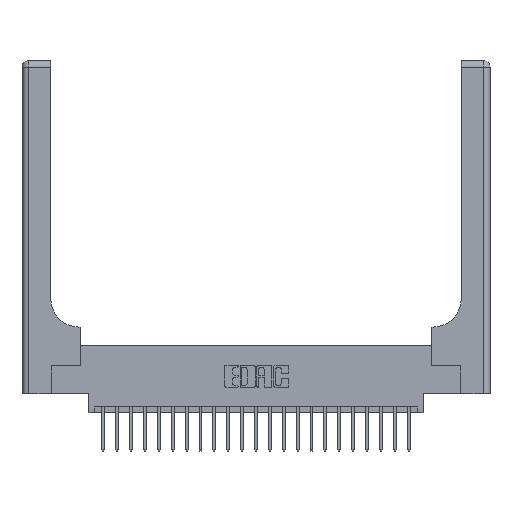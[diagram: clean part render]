
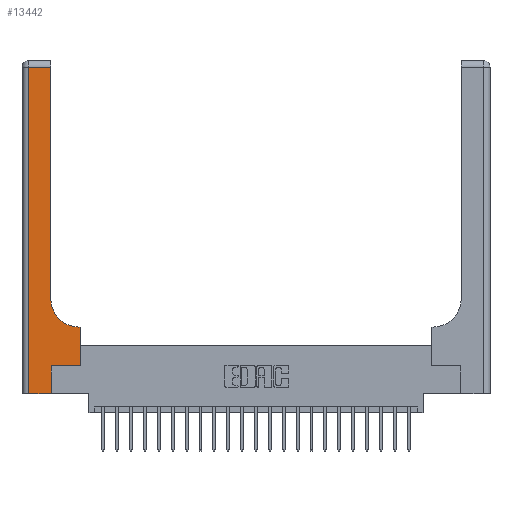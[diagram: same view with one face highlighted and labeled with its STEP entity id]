
A CAD part, top view. The second image highlights one B-rep face of the part: STEP entity #13442.
In plain terms, the highlighted planar face has unit normal (0, 0, 1).
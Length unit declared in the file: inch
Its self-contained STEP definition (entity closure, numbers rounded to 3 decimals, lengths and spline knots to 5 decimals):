
#214 = CARTESIAN_POINT ( 'NONE',  ( 0.528, 0.25, 0.37 ) ) ;
#1040 = FACE_OUTER_BOUND ( 'NONE', #20236, .T. ) ;
#1073 = LINE ( 'NONE', #2807, #9994 ) ;
#1435 = DIRECTION ( 'NONE',  ( -1., 0., 0. ) ) ;
#1828 = VERTEX_POINT ( 'NONE', #9750 ) ;
#1956 = LINE ( 'NONE', #16306, #15564 ) ;
#2047 = EDGE_CURVE ( 'NONE', #22063, #15384, #9610, .T. ) ;
#2102 = ORIENTED_EDGE ( 'NONE', *, *, #2047, .T. ) ;
#2450 = CARTESIAN_POINT ( 'NONE',  ( 0.06, 3., 0.37 ) ) ;
#2740 = VERTEX_POINT ( 'NONE', #214 ) ;
#2807 = CARTESIAN_POINT ( 'NONE',  ( 0., 0., 0.37 ) ) ;
#3266 = VERTEX_POINT ( 'NONE', #7070 ) ;
#3744 = VERTEX_POINT ( 'NONE', #4850 ) ;
#3780 = LINE ( 'NONE', #5751, #12620 ) ;
#4211 = AXIS2_PLACEMENT_3D ( 'NONE', #6793, #19141, #8558 ) ;
#4232 = DIRECTION ( 'NONE',  ( 0., -1., 0. ) ) ;
#4833 = CARTESIAN_POINT ( 'NONE',  ( 0.265, 0., 0.37 ) ) ;
#4850 = CARTESIAN_POINT ( 'NONE',  ( 0.06, 2.94, 0.37 ) ) ;
#4902 = VECTOR ( 'NONE', #10598, 39.37008 ) ;
#5751 = CARTESIAN_POINT ( 'NONE',  ( 0.528, 0.25, 0.37 ) ) ;
#6172 = ORIENTED_EDGE ( 'NONE', *, *, #21710, .T. ) ;
#6442 = DIRECTION ( 'NONE',  ( 1., 0., 0. ) ) ;
#6793 = CARTESIAN_POINT ( 'NONE',  ( 0., 3., 0.37 ) ) ;
#7023 = VECTOR ( 'NONE', #19616, 39.37008 ) ;
#7070 = CARTESIAN_POINT ( 'NONE',  ( 0.06, 0., 0.37 ) ) ;
#7123 = ORIENTED_EDGE ( 'NONE', *, *, #18477, .T. ) ;
#7525 = DIRECTION ( 'NONE',  ( 0., 1., 0. ) ) ;
#7563 = DIRECTION ( 'NONE',  ( 0., 0., -1. ) ) ;
#8558 = DIRECTION ( 'NONE',  ( -1., 0., 0. ) ) ;
#8615 = VECTOR ( 'NONE', #18991, 39.37008 ) ;
#8810 = CARTESIAN_POINT ( 'NONE',  ( 0.26, 3., 0.37 ) ) ;
#9063 = LINE ( 'NONE', #2450, #15463 ) ;
#9108 = ORIENTED_EDGE ( 'NONE', *, *, #11271, .T. ) ;
#9610 = LINE ( 'NONE', #8810, #4902 ) ;
#9750 = CARTESIAN_POINT ( 'NONE',  ( 0.528, 0.6, 0.37 ) ) ;
#9994 = VECTOR ( 'NONE', #6442, 39.37008 ) ;
#10598 = DIRECTION ( 'NONE',  ( 0., 1., 0. ) ) ;
#10724 = CARTESIAN_POINT ( 'NONE',  ( 0.26, 0.85, 0.37 ) ) ;
#11271 = EDGE_CURVE ( 'NONE', #15910, #22063, #18858, .T. ) ;
#11531 = EDGE_CURVE ( 'NONE', #17771, #12057, #17486, .T. ) ;
#12057 = VERTEX_POINT ( 'NONE', #14979 ) ;
#12078 = CARTESIAN_POINT ( 'NONE',  ( 0.26, 0.6, 0.37 ) ) ;
#12620 = VECTOR ( 'NONE', #7525, 39.37008 ) ;
#13442 = ADVANCED_FACE ( 'NONE', ( #1040 ), #13847, .F. ) ;
#13847 = PLANE ( 'NONE',  #4211 ) ;
#14416 = CARTESIAN_POINT ( 'NONE',  ( 0.265, 0., 0.37 ) ) ;
#14979 = CARTESIAN_POINT ( 'NONE',  ( 0.265, 0.25, 0.37 ) ) ;
#15217 = ORIENTED_EDGE ( 'NONE', *, *, #21300, .T. ) ;
#15305 = AXIS2_PLACEMENT_3D ( 'NONE', #18157, #7563, #19887 ) ;
#15384 = VERTEX_POINT ( 'NONE', #21439 ) ;
#15463 = VECTOR ( 'NONE', #4232, 39.37008 ) ;
#15564 = VECTOR ( 'NONE', #18070, 39.37008 ) ;
#15910 = VERTEX_POINT ( 'NONE', #21348 ) ;
#16306 = CARTESIAN_POINT ( 'NONE',  ( 0., 2.94, 0.37 ) ) ;
#16868 = LINE ( 'NONE', #12078, #17964 ) ;
#16917 = ORIENTED_EDGE ( 'NONE', *, *, #19244, .T. ) ;
#17486 = LINE ( 'NONE', #4833, #8615 ) ;
#17745 = EDGE_CURVE ( 'NONE', #12057, #2740, #21077, .T. ) ;
#17771 = VERTEX_POINT ( 'NONE', #14416 ) ;
#17870 = CARTESIAN_POINT ( 'NONE',  ( 0.265, 0.25, 0.37 ) ) ;
#17964 = VECTOR ( 'NONE', #1435, 39.37008 ) ;
#18070 = DIRECTION ( 'NONE',  ( -1., 0., 0. ) ) ;
#18157 = CARTESIAN_POINT ( 'NONE',  ( 0.51, 0.85, 0.37 ) ) ;
#18477 = EDGE_CURVE ( 'NONE', #15384, #3744, #1956, .T. ) ;
#18698 = ORIENTED_EDGE ( 'NONE', *, *, #17745, .T. ) ;
#18858 = CIRCLE ( 'NONE', #15305, 0.25 ) ;
#18991 = DIRECTION ( 'NONE',  ( 0., 1., 0. ) ) ;
#19141 = DIRECTION ( 'NONE',  ( 0., 0., -1. ) ) ;
#19244 = EDGE_CURVE ( 'NONE', #3266, #17771, #1073, .T. ) ;
#19616 = DIRECTION ( 'NONE',  ( 1., 0., 0. ) ) ;
#19887 = DIRECTION ( 'NONE',  ( 1., 0., 0. ) ) ;
#20236 = EDGE_LOOP ( 'NONE', ( #2102, #7123, #6172, #16917, #21125, #18698, #22711, #15217, #9108 ) ) ;
#21077 = LINE ( 'NONE', #17870, #7023 ) ;
#21125 = ORIENTED_EDGE ( 'NONE', *, *, #11531, .T. ) ;
#21300 = EDGE_CURVE ( 'NONE', #1828, #15910, #16868, .T. ) ;
#21348 = CARTESIAN_POINT ( 'NONE',  ( 0.51, 0.6, 0.37 ) ) ;
#21439 = CARTESIAN_POINT ( 'NONE',  ( 0.26, 2.94, 0.37 ) ) ;
#21710 = EDGE_CURVE ( 'NONE', #3744, #3266, #9063, .T. ) ;
#22063 = VERTEX_POINT ( 'NONE', #10724 ) ;
#22711 = ORIENTED_EDGE ( 'NONE', *, *, #22731, .T. ) ;
#22731 = EDGE_CURVE ( 'NONE', #2740, #1828, #3780, .T. ) ;
